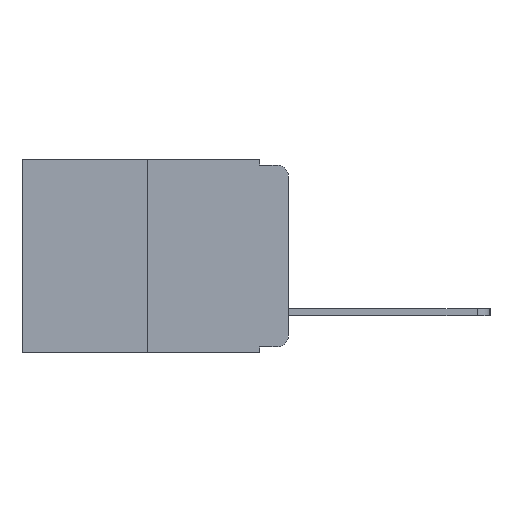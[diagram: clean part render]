
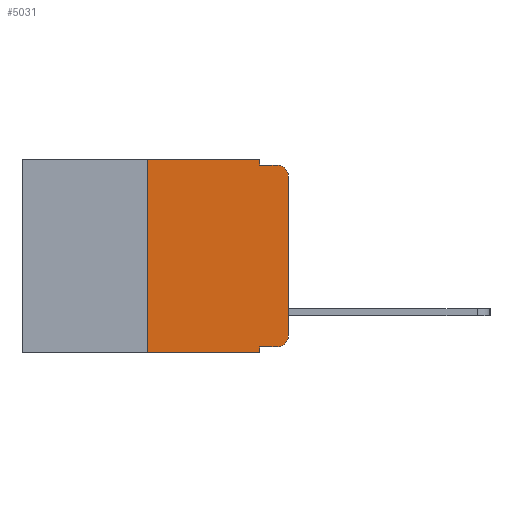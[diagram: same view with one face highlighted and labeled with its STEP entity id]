
A CAD part, left-side view. The second image highlights one B-rep face of the part: STEP entity #5031.
In plain terms, the highlighted planar face has unit normal (-1, 0, 0).
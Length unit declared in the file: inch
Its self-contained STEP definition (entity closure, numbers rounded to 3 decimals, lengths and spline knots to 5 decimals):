
#128 = CARTESIAN_POINT ( 'NONE',  ( 0., 0.473, 0. ) ) ;
#313 = EDGE_CURVE ( 'NONE', #8340, #21473, #14763, .T. ) ;
#561 = DIRECTION ( 'NONE',  ( 0., 0., -1. ) ) ;
#620 = VERTEX_POINT ( 'NONE', #21046 ) ;
#988 = ORIENTED_EDGE ( 'NONE', *, *, #10652, .T. ) ;
#1233 = CARTESIAN_POINT ( 'NONE',  ( 0., 0.051, -0.333 ) ) ;
#1573 = EDGE_CURVE ( 'NONE', #21473, #21866, #2595, .T. ) ;
#1603 = DIRECTION ( 'NONE',  ( 0., -1., 0. ) ) ;
#2526 = VECTOR ( 'NONE', #561, 39.37008 ) ;
#2589 = CARTESIAN_POINT ( 'NONE',  ( 0., 0., 0. ) ) ;
#2595 = CIRCLE ( 'NONE', #17495, 0.02 ) ;
#2699 = VECTOR ( 'NONE', #5099, 39.37008 ) ;
#3296 = CARTESIAN_POINT ( 'NONE',  ( 0., 0.051, 0. ) ) ;
#3500 = VECTOR ( 'NONE', #8596, 39.37008 ) ;
#3817 = LINE ( 'NONE', #3296, #2699 ) ;
#4469 = ORIENTED_EDGE ( 'NONE', *, *, #1573, .T. ) ;
#4530 = DIRECTION ( 'NONE',  ( 0., -1., 0. ) ) ;
#4634 = VERTEX_POINT ( 'NONE', #19253 ) ;
#4723 = ORIENTED_EDGE ( 'NONE', *, *, #17295, .F. ) ;
#4920 = CARTESIAN_POINT ( 'NONE',  ( 0., 0.051, -0.01 ) ) ;
#5031 = ADVANCED_FACE ( 'NONE', ( #6963 ), #15316, .F. ) ;
#5099 = DIRECTION ( 'NONE',  ( 0., 0., -1. ) ) ;
#5832 = ORIENTED_EDGE ( 'NONE', *, *, #19627, .F. ) ;
#5845 = CARTESIAN_POINT ( 'NONE',  ( 0., 0., -0.313 ) ) ;
#6095 = EDGE_LOOP ( 'NONE', ( #9330, #988, #5832, #11323, #4723, #14328, #18707, #11894, #17949, #4469 ) ) ;
#6157 = VERTEX_POINT ( 'NONE', #8659 ) ;
#6407 = DIRECTION ( 'NONE',  ( 1., 0., 0. ) ) ;
#6756 = CIRCLE ( 'NONE', #17832, 0.02 ) ;
#6791 = CARTESIAN_POINT ( 'NONE',  ( 0., 0.25, 0. ) ) ;
#6796 = VERTEX_POINT ( 'NONE', #7526 ) ;
#6918 = EDGE_CURVE ( 'NONE', #21866, #16216, #13159, .T. ) ;
#6963 = FACE_OUTER_BOUND ( 'NONE', #6095, .T. ) ;
#7355 = LINE ( 'NONE', #11553, #2526 ) ;
#7526 = CARTESIAN_POINT ( 'NONE',  ( 0., 0.25, -0.343 ) ) ;
#7586 = LINE ( 'NONE', #128, #20748 ) ;
#8007 = DIRECTION ( 'NONE',  ( 0., 0., 1. ) ) ;
#8340 = VERTEX_POINT ( 'NONE', #12786 ) ;
#8596 = DIRECTION ( 'NONE',  ( 0., -1., 0. ) ) ;
#8634 = EDGE_CURVE ( 'NONE', #6796, #4634, #14938, .T. ) ;
#8659 = CARTESIAN_POINT ( 'NONE',  ( 0., 0.051, 0. ) ) ;
#8821 = DIRECTION ( 'NONE',  ( -1., 0., 0. ) ) ;
#8911 = CARTESIAN_POINT ( 'NONE',  ( 0., 0.473, -0.343 ) ) ;
#9330 = ORIENTED_EDGE ( 'NONE', *, *, #6918, .T. ) ;
#9890 = EDGE_CURVE ( 'NONE', #6157, #9983, #7355, .T. ) ;
#9983 = VERTEX_POINT ( 'NONE', #21719 ) ;
#10155 = VECTOR ( 'NONE', #4530, 39.37008 ) ;
#10335 = VECTOR ( 'NONE', #15713, 39.37008 ) ;
#10652 = EDGE_CURVE ( 'NONE', #16216, #620, #6756, .T. ) ;
#11323 = ORIENTED_EDGE ( 'NONE', *, *, #9890, .F. ) ;
#11553 = CARTESIAN_POINT ( 'NONE',  ( 0., 0.051, 0. ) ) ;
#11806 = EDGE_CURVE ( 'NONE', #8340, #17498, #3817, .T. ) ;
#11894 = ORIENTED_EDGE ( 'NONE', *, *, #11806, .F. ) ;
#12786 = CARTESIAN_POINT ( 'NONE',  ( 0., 0.051, -0.333 ) ) ;
#13159 = LINE ( 'NONE', #2589, #17101 ) ;
#13968 = DIRECTION ( 'NONE',  ( -1., 0., 0. ) ) ;
#14328 = ORIENTED_EDGE ( 'NONE', *, *, #8634, .F. ) ;
#14611 = DIRECTION ( 'NONE',  ( 0., -1., 0. ) ) ;
#14763 = LINE ( 'NONE', #1233, #10155 ) ;
#14938 = LINE ( 'NONE', #6791, #10335 ) ;
#15316 = PLANE ( 'NONE',  #21912 ) ;
#15713 = DIRECTION ( 'NONE',  ( 0., 0., 1. ) ) ;
#16216 = VERTEX_POINT ( 'NONE', #16320 ) ;
#16320 = CARTESIAN_POINT ( 'NONE',  ( 0., 0., -0.03 ) ) ;
#16450 = VECTOR ( 'NONE', #1603, 39.37008 ) ;
#16953 = CARTESIAN_POINT ( 'NONE',  ( 0., 0.473, 0. ) ) ;
#16954 = LINE ( 'NONE', #8911, #16450 ) ;
#17101 = VECTOR ( 'NONE', #8007, 39.37008 ) ;
#17295 = EDGE_CURVE ( 'NONE', #4634, #6157, #7586, .T. ) ;
#17495 = AXIS2_PLACEMENT_3D ( 'NONE', #19120, #13968, #22031 ) ;
#17498 = VERTEX_POINT ( 'NONE', #21619 ) ;
#17832 = AXIS2_PLACEMENT_3D ( 'NONE', #19039, #8821, #20692 ) ;
#17949 = ORIENTED_EDGE ( 'NONE', *, *, #313, .T. ) ;
#18593 = DIRECTION ( 'NONE',  ( 0., 0., -1. ) ) ;
#18707 = ORIENTED_EDGE ( 'NONE', *, *, #20555, .T. ) ;
#19039 = CARTESIAN_POINT ( 'NONE',  ( 0., 0.02, -0.03 ) ) ;
#19120 = CARTESIAN_POINT ( 'NONE',  ( 0., 0.02, -0.313 ) ) ;
#19253 = CARTESIAN_POINT ( 'NONE',  ( 0., 0.25, 0. ) ) ;
#19627 = EDGE_CURVE ( 'NONE', #9983, #620, #21926, .T. ) ;
#20555 = EDGE_CURVE ( 'NONE', #6796, #17498, #16954, .T. ) ;
#20692 = DIRECTION ( 'NONE',  ( 0., 0., -1. ) ) ;
#20748 = VECTOR ( 'NONE', #14611, 39.37008 ) ;
#21046 = CARTESIAN_POINT ( 'NONE',  ( 0., 0.02, -0.01 ) ) ;
#21473 = VERTEX_POINT ( 'NONE', #22400 ) ;
#21619 = CARTESIAN_POINT ( 'NONE',  ( 0., 0.051, -0.343 ) ) ;
#21719 = CARTESIAN_POINT ( 'NONE',  ( 0., 0.051, -0.01 ) ) ;
#21866 = VERTEX_POINT ( 'NONE', #5845 ) ;
#21912 = AXIS2_PLACEMENT_3D ( 'NONE', #16953, #6407, #18593 ) ;
#21926 = LINE ( 'NONE', #4920, #3500 ) ;
#22031 = DIRECTION ( 'NONE',  ( 0., 0., -1. ) ) ;
#22400 = CARTESIAN_POINT ( 'NONE',  ( 0., 0.02, -0.333 ) ) ;
